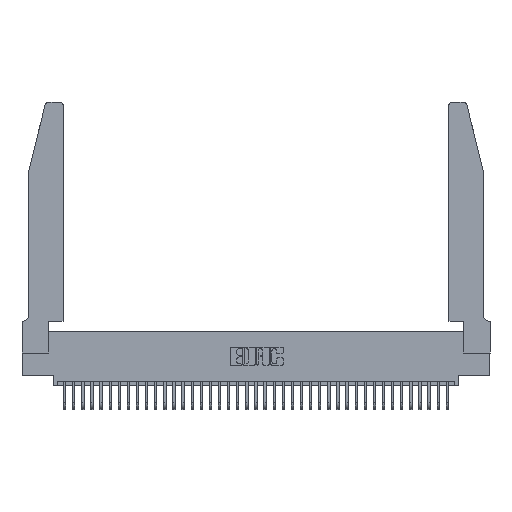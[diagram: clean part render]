
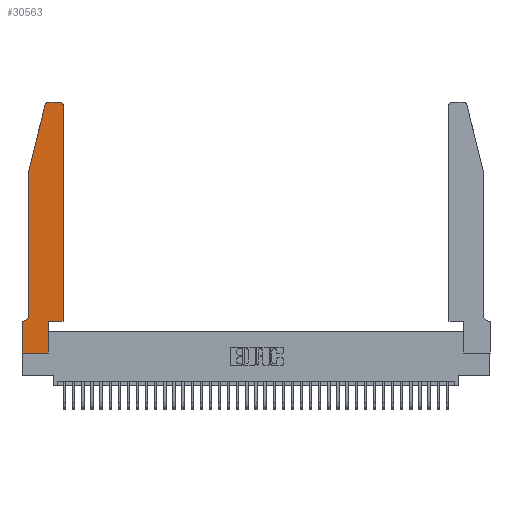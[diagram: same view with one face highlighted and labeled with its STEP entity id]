
A CAD part, top view. The second image highlights one B-rep face of the part: STEP entity #30563.
In plain terms, the highlighted planar face has unit normal (0, 0, 1).
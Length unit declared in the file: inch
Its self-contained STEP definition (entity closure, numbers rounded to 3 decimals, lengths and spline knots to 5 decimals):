
#105 = EDGE_CURVE ( 'NONE', #16642, #14556, #15248, .T. ) ;
#555 = LINE ( 'NONE', #34734, #7381 ) ;
#678 = VECTOR ( 'NONE', #31490, 39.37008 ) ;
#1815 = CARTESIAN_POINT ( 'NONE',  ( 0.0755, 2., 0.37 ) ) ;
#2619 = EDGE_LOOP ( 'NONE', ( #37134, #5811, #24337, #24808, #36134, #22500, #28045, #24198, #33826, #4392, #10906, #4061 ) ) ;
#2762 = VERTEX_POINT ( 'NONE', #10835 ) ;
#3209 = VECTOR ( 'NONE', #8167, 39.37008 ) ;
#4061 = ORIENTED_EDGE ( 'NONE', *, *, #7948, .T. ) ;
#4392 = ORIENTED_EDGE ( 'NONE', *, *, #21749, .T. ) ;
#4440 = LINE ( 'NONE', #30159, #12101 ) ;
#5173 = CARTESIAN_POINT ( 'NONE',  ( 0.284, 2.75, 0.37 ) ) ;
#5192 = DIRECTION ( 'NONE',  ( 0., 0., 1. ) ) ;
#5811 = ORIENTED_EDGE ( 'NONE', *, *, #14804, .T. ) ;
#5986 = AXIS2_PLACEMENT_3D ( 'NONE', #27199, #10052, #30068 ) ;
#6734 = CIRCLE ( 'NONE', #24407, 0.03 ) ;
#7059 = DIRECTION ( 'NONE',  ( 1., 0., 0. ) ) ;
#7381 = VECTOR ( 'NONE', #23219, 39.37008 ) ;
#7566 = VERTEX_POINT ( 'NONE', #5173 ) ;
#7948 = EDGE_CURVE ( 'NONE', #31988, #11439, #14096, .T. ) ;
#8167 = DIRECTION ( 'NONE',  ( -1., 0., 0. ) ) ;
#10052 = DIRECTION ( 'NONE',  ( 0., 0., 1. ) ) ;
#10178 = EDGE_CURVE ( 'NONE', #2762, #16147, #30322, .T. ) ;
#10312 = DIRECTION ( 'NONE',  ( -0.239, -0.971, 0. ) ) ;
#10807 = DIRECTION ( 'NONE',  ( 1., 0., 0. ) ) ;
#10835 = CARTESIAN_POINT ( 'NONE',  ( 0.2865, 0., 0.37 ) ) ;
#10906 = ORIENTED_EDGE ( 'NONE', *, *, #20181, .T. ) ;
#11417 = VECTOR ( 'NONE', #10807, 39.37008 ) ;
#11439 = VERTEX_POINT ( 'NONE', #17419 ) ;
#12101 = VECTOR ( 'NONE', #13051, 39.37008 ) ;
#12107 = CARTESIAN_POINT ( 'NONE',  ( 0., 0., 0.37 ) ) ;
#12159 = DIRECTION ( 'NONE',  ( -1., 0., 0. ) ) ;
#12680 = AXIS2_PLACEMENT_3D ( 'NONE', #17933, #16459, #12159 ) ;
#12754 = VERTEX_POINT ( 'NONE', #12943 ) ;
#12943 = CARTESIAN_POINT ( 'NONE',  ( 0.4505, 0.35, 0.37 ) ) ;
#13051 = DIRECTION ( 'NONE',  ( 0., 1., 0. ) ) ;
#13289 = DIRECTION ( 'NONE',  ( 0., 0., 1. ) ) ;
#13696 = EDGE_CURVE ( 'NONE', #33813, #16642, #19851, .T. ) ;
#13705 = VERTEX_POINT ( 'NONE', #21618 ) ;
#14096 = CIRCLE ( 'NONE', #5986, 0.03 ) ;
#14556 = VERTEX_POINT ( 'NONE', #17943 ) ;
#14804 = EDGE_CURVE ( 'NONE', #7566, #13705, #6734, .T. ) ;
#14998 = LINE ( 'NONE', #12107, #22573 ) ;
#15248 = CIRCLE ( 'NONE', #12680, 0.07 ) ;
#16147 = VERTEX_POINT ( 'NONE', #20989 ) ;
#16426 = EDGE_CURVE ( 'NONE', #34103, #2762, #19957, .T. ) ;
#16459 = DIRECTION ( 'NONE',  ( 0., 0., -1. ) ) ;
#16642 = VERTEX_POINT ( 'NONE', #32057 ) ;
#17419 = CARTESIAN_POINT ( 'NONE',  ( 0.4205, 2.75, 0.37 ) ) ;
#17844 = EDGE_CURVE ( 'NONE', #36319, #34103, #14998, .T. ) ;
#17933 = CARTESIAN_POINT ( 'NONE',  ( 0.0055, 0.42, 0.37 ) ) ;
#17943 = CARTESIAN_POINT ( 'NONE',  ( 0.0055, 0.35, 0.37 ) ) ;
#18195 = EDGE_CURVE ( 'NONE', #14556, #36319, #19442, .T. ) ;
#18763 = DIRECTION ( 'NONE',  ( 0., -1., 0. ) ) ;
#19442 = LINE ( 'NONE', #25318, #3209 ) ;
#19851 = LINE ( 'NONE', #35871, #26518 ) ;
#19957 = LINE ( 'NONE', #36577, #11417 ) ;
#20138 = CARTESIAN_POINT ( 'NONE',  ( 0.2865, 0.35, 0.37 ) ) ;
#20181 = EDGE_CURVE ( 'NONE', #12754, #31988, #4440, .T. ) ;
#20296 = CARTESIAN_POINT ( 'NONE',  ( 0.4505, 2.72, 0.37 ) ) ;
#20989 = CARTESIAN_POINT ( 'NONE',  ( 0.2865, 0.35, 0.37 ) ) ;
#21618 = CARTESIAN_POINT ( 'NONE',  ( 0.25487, 2.72718, 0.37 ) ) ;
#21660 = AXIS2_PLACEMENT_3D ( 'NONE', #22385, #5192, #25243 ) ;
#21749 = EDGE_CURVE ( 'NONE', #16147, #12754, #30604, .T. ) ;
#21879 = EDGE_CURVE ( 'NONE', #13705, #33813, #33768, .T. ) ;
#22385 = CARTESIAN_POINT ( 'NONE',  ( 0., 0.35, 0.37 ) ) ;
#22500 = ORIENTED_EDGE ( 'NONE', *, *, #18195, .T. ) ;
#22573 = VECTOR ( 'NONE', #26211, 39.37008 ) ;
#23219 = DIRECTION ( 'NONE',  ( -1., 0., 0. ) ) ;
#23913 = VECTOR ( 'NONE', #7059, 39.37008 ) ;
#24198 = ORIENTED_EDGE ( 'NONE', *, *, #16426, .T. ) ;
#24219 = FACE_OUTER_BOUND ( 'NONE', #2619, .T. ) ;
#24337 = ORIENTED_EDGE ( 'NONE', *, *, #21879, .T. ) ;
#24407 = AXIS2_PLACEMENT_3D ( 'NONE', #30393, #13289, #33311 ) ;
#24808 = ORIENTED_EDGE ( 'NONE', *, *, #13696, .T. ) ;
#25243 = DIRECTION ( 'NONE',  ( 1., 0., 0. ) ) ;
#25318 = CARTESIAN_POINT ( 'NONE',  ( 0.0755, 0.35, 0.37 ) ) ;
#26099 = VECTOR ( 'NONE', #10312, 39.37008 ) ;
#26211 = DIRECTION ( 'NONE',  ( 0., -1., 0. ) ) ;
#26518 = VECTOR ( 'NONE', #18763, 39.37008 ) ;
#26718 = CARTESIAN_POINT ( 'NONE',  ( 0.0755, 2., 0.37 ) ) ;
#27199 = CARTESIAN_POINT ( 'NONE',  ( 0.4205, 2.72, 0.37 ) ) ;
#27280 = EDGE_CURVE ( 'NONE', #11439, #7566, #555, .T. ) ;
#28045 = ORIENTED_EDGE ( 'NONE', *, *, #17844, .T. ) ;
#30068 = DIRECTION ( 'NONE',  ( 1., 0., 0. ) ) ;
#30159 = CARTESIAN_POINT ( 'NONE',  ( 0.4505, 0.35, 0.37 ) ) ;
#30322 = LINE ( 'NONE', #20138, #678 ) ;
#30393 = CARTESIAN_POINT ( 'NONE',  ( 0.284, 2.72, 0.37 ) ) ;
#30563 = ADVANCED_FACE ( 'NONE', ( #24219 ), #36628, .T. ) ;
#30604 = LINE ( 'NONE', #35607, #23913 ) ;
#31490 = DIRECTION ( 'NONE',  ( 0., 1., 0. ) ) ;
#31813 = CARTESIAN_POINT ( 'NONE',  ( 0., 0., 0.37 ) ) ;
#31988 = VERTEX_POINT ( 'NONE', #20296 ) ;
#32057 = CARTESIAN_POINT ( 'NONE',  ( 0.0755, 0.42, 0.37 ) ) ;
#33311 = DIRECTION ( 'NONE',  ( 1., 0., 0. ) ) ;
#33768 = LINE ( 'NONE', #1815, #26099 ) ;
#33813 = VERTEX_POINT ( 'NONE', #26718 ) ;
#33826 = ORIENTED_EDGE ( 'NONE', *, *, #10178, .T. ) ;
#34103 = VERTEX_POINT ( 'NONE', #31813 ) ;
#34734 = CARTESIAN_POINT ( 'NONE',  ( 0.2605, 2.75, 0.37 ) ) ;
#35607 = CARTESIAN_POINT ( 'NONE',  ( 0.4505, 0.35, 0.37 ) ) ;
#35871 = CARTESIAN_POINT ( 'NONE',  ( 0.0755, 2., 0.37 ) ) ;
#36134 = ORIENTED_EDGE ( 'NONE', *, *, #105, .T. ) ;
#36319 = VERTEX_POINT ( 'NONE', #36912 ) ;
#36577 = CARTESIAN_POINT ( 'NONE',  ( 0., 0., 0.37 ) ) ;
#36628 = PLANE ( 'NONE',  #21660 ) ;
#36912 = CARTESIAN_POINT ( 'NONE',  ( 0., 0.35, 0.37 ) ) ;
#37134 = ORIENTED_EDGE ( 'NONE', *, *, #27280, .T. ) ;
